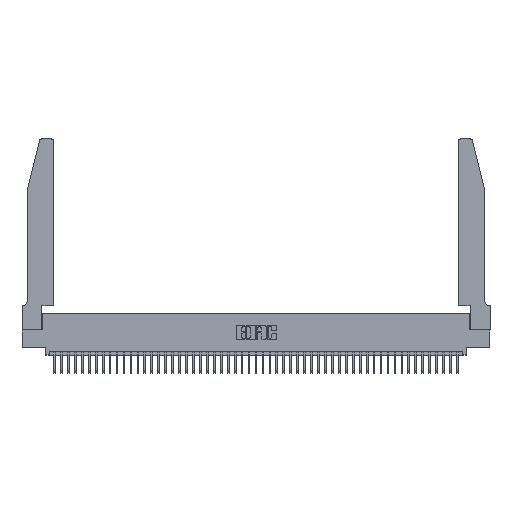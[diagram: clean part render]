
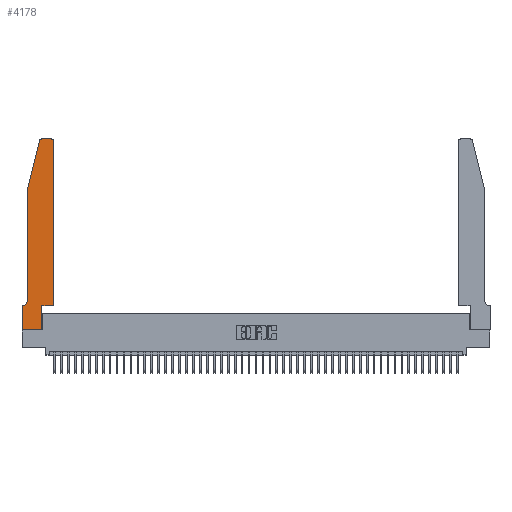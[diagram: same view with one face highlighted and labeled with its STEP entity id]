
A CAD part, top view. The second image highlights one B-rep face of the part: STEP entity #4178.
In plain terms, the highlighted planar face has unit normal (0, 0, 1).
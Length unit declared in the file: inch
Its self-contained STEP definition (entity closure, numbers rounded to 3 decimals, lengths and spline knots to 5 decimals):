
#5 = EDGE_LOOP ( 'NONE', ( #31108, #38971, #48633, #9396, #12701, #38850, #44825, #49659, #22916, #21874, #20541, #32753 ) ) ;
#1253 = VERTEX_POINT ( 'NONE', #48712 ) ;
#2338 = DIRECTION ( 'NONE',  ( 0., 0., -1. ) ) ;
#3318 = CARTESIAN_POINT ( 'NONE',  ( 0.0755, 2., 0.37 ) ) ;
#3496 = AXIS2_PLACEMENT_3D ( 'NONE', #46667, #46176, #20033 ) ;
#4178 = ADVANCED_FACE ( 'NONE', ( #18619 ), #47686, .T. ) ;
#4203 = DIRECTION ( 'NONE',  ( 0., -1., 0. ) ) ;
#4557 = VERTEX_POINT ( 'NONE', #26676 ) ;
#5245 = CARTESIAN_POINT ( 'NONE',  ( 0.25487, 2.72718, 0.37 ) ) ;
#5362 = LINE ( 'NONE', #15091, #50573 ) ;
#5391 = VERTEX_POINT ( 'NONE', #5245 ) ;
#5493 = CARTESIAN_POINT ( 'NONE',  ( 0., 0., 0.37 ) ) ;
#5517 = EDGE_CURVE ( 'NONE', #38527, #18075, #36779, .T. ) ;
#5591 = VECTOR ( 'NONE', #48440, 39.37008 ) ;
#6948 = LINE ( 'NONE', #45353, #34970 ) ;
#7301 = EDGE_CURVE ( 'NONE', #40261, #5391, #34787, .T. ) ;
#8132 = CARTESIAN_POINT ( 'NONE',  ( 0.0755, 2., 0.37 ) ) ;
#8458 = CARTESIAN_POINT ( 'NONE',  ( 0., 0.35, 0.37 ) ) ;
#9337 = VECTOR ( 'NONE', #25352, 39.37008 ) ;
#9396 = ORIENTED_EDGE ( 'NONE', *, *, #14602, .T. ) ;
#9519 = DIRECTION ( 'NONE',  ( -1., 0., 0. ) ) ;
#9538 = VECTOR ( 'NONE', #47108, 39.37008 ) ;
#10536 = DIRECTION ( 'NONE',  ( 1., 0., 0. ) ) ;
#12701 = ORIENTED_EDGE ( 'NONE', *, *, #5517, .T. ) ;
#13118 = LINE ( 'NONE', #46714, #46727 ) ;
#14443 = CARTESIAN_POINT ( 'NONE',  ( 0.284, 2.75, 0.37 ) ) ;
#14602 = EDGE_CURVE ( 'NONE', #28823, #38527, #18881, .T. ) ;
#15091 = CARTESIAN_POINT ( 'NONE',  ( 0.0755, 2., 0.37 ) ) ;
#15298 = LINE ( 'NONE', #22449, #39741 ) ;
#15403 = LINE ( 'NONE', #21926, #9337 ) ;
#15784 = VECTOR ( 'NONE', #4203, 39.37008 ) ;
#17063 = CARTESIAN_POINT ( 'NONE',  ( 0.4505, 2.72, 0.37 ) ) ;
#17135 = EDGE_CURVE ( 'NONE', #18075, #33438, #28187, .T. ) ;
#17838 = DIRECTION ( 'NONE',  ( 1., 0., 0. ) ) ;
#18075 = VERTEX_POINT ( 'NONE', #36444 ) ;
#18619 = FACE_OUTER_BOUND ( 'NONE', #5, .T. ) ;
#18881 = LINE ( 'NONE', #8132, #15784 ) ;
#18951 = CARTESIAN_POINT ( 'NONE',  ( 0.0755, 0.35, 0.37 ) ) ;
#19025 = AXIS2_PLACEMENT_3D ( 'NONE', #8458, #24304, #28271 ) ;
#20033 = DIRECTION ( 'NONE',  ( 1., 0., 0. ) ) ;
#20541 = ORIENTED_EDGE ( 'NONE', *, *, #28687, .T. ) ;
#21041 = VERTEX_POINT ( 'NONE', #5493 ) ;
#21874 = ORIENTED_EDGE ( 'NONE', *, *, #42524, .T. ) ;
#21926 = CARTESIAN_POINT ( 'NONE',  ( 0.4505, 0.35, 0.37 ) ) ;
#21927 = EDGE_CURVE ( 'NONE', #21041, #1253, #6948, .T. ) ;
#22205 = CIRCLE ( 'NONE', #3496, 0.03 ) ;
#22449 = CARTESIAN_POINT ( 'NONE',  ( 0.2605, 2.75, 0.37 ) ) ;
#22916 = ORIENTED_EDGE ( 'NONE', *, *, #46537, .T. ) ;
#23075 = AXIS2_PLACEMENT_3D ( 'NONE', #44815, #44995, #17838 ) ;
#24304 = DIRECTION ( 'NONE',  ( 0., 0., 1. ) ) ;
#24861 = CARTESIAN_POINT ( 'NONE',  ( 0.4505, 0.35, 0.37 ) ) ;
#25035 = CARTESIAN_POINT ( 'NONE',  ( 0.0755, 0.42, 0.37 ) ) ;
#25352 = DIRECTION ( 'NONE',  ( 0., 1., 0. ) ) ;
#25389 = LINE ( 'NONE', #39883, #9538 ) ;
#26562 = DIRECTION ( 'NONE',  ( -0.239, -0.971, 0. ) ) ;
#26676 = CARTESIAN_POINT ( 'NONE',  ( 0.2865, 0.35, 0.37 ) ) ;
#28187 = LINE ( 'NONE', #18951, #45869 ) ;
#28271 = DIRECTION ( 'NONE',  ( 1., 0., 0. ) ) ;
#28687 = EDGE_CURVE ( 'NONE', #42014, #42179, #15403, .T. ) ;
#28823 = VERTEX_POINT ( 'NONE', #3318 ) ;
#29158 = CARTESIAN_POINT ( 'NONE',  ( 0.0055, 0.42, 0.37 ) ) ;
#31108 = ORIENTED_EDGE ( 'NONE', *, *, #42598, .T. ) ;
#32753 = ORIENTED_EDGE ( 'NONE', *, *, #38944, .T. ) ;
#33438 = VERTEX_POINT ( 'NONE', #47121 ) ;
#33977 = EDGE_CURVE ( 'NONE', #33438, #21041, #13118, .T. ) ;
#34699 = VERTEX_POINT ( 'NONE', #46305 ) ;
#34787 = CIRCLE ( 'NONE', #23075, 0.03 ) ;
#34970 = VECTOR ( 'NONE', #10536, 39.37008 ) ;
#35912 = EDGE_CURVE ( 'NONE', #5391, #28823, #5362, .T. ) ;
#36207 = AXIS2_PLACEMENT_3D ( 'NONE', #29158, #2338, #9519 ) ;
#36444 = CARTESIAN_POINT ( 'NONE',  ( 0.0055, 0.35, 0.37 ) ) ;
#36779 = CIRCLE ( 'NONE', #36207, 0.07 ) ;
#38527 = VERTEX_POINT ( 'NONE', #25035 ) ;
#38850 = ORIENTED_EDGE ( 'NONE', *, *, #17135, .T. ) ;
#38944 = EDGE_CURVE ( 'NONE', #42179, #34699, #22205, .T. ) ;
#38971 = ORIENTED_EDGE ( 'NONE', *, *, #7301, .T. ) ;
#39741 = VECTOR ( 'NONE', #45174, 39.37008 ) ;
#39883 = CARTESIAN_POINT ( 'NONE',  ( 0.2865, 0.35, 0.37 ) ) ;
#40261 = VERTEX_POINT ( 'NONE', #14443 ) ;
#41446 = CARTESIAN_POINT ( 'NONE',  ( 0.4505, 0.35, 0.37 ) ) ;
#42014 = VERTEX_POINT ( 'NONE', #41446 ) ;
#42179 = VERTEX_POINT ( 'NONE', #17063 ) ;
#42524 = EDGE_CURVE ( 'NONE', #4557, #42014, #48365, .T. ) ;
#42598 = EDGE_CURVE ( 'NONE', #34699, #40261, #15298, .T. ) ;
#44815 = CARTESIAN_POINT ( 'NONE',  ( 0.284, 2.72, 0.37 ) ) ;
#44825 = ORIENTED_EDGE ( 'NONE', *, *, #33977, .T. ) ;
#44995 = DIRECTION ( 'NONE',  ( 0., 0., 1. ) ) ;
#45174 = DIRECTION ( 'NONE',  ( -1., 0., 0. ) ) ;
#45353 = CARTESIAN_POINT ( 'NONE',  ( 0., 0., 0.37 ) ) ;
#45869 = VECTOR ( 'NONE', #45936, 39.37008 ) ;
#45936 = DIRECTION ( 'NONE',  ( -1., 0., 0. ) ) ;
#46176 = DIRECTION ( 'NONE',  ( 0., 0., 1. ) ) ;
#46305 = CARTESIAN_POINT ( 'NONE',  ( 0.4205, 2.75, 0.37 ) ) ;
#46537 = EDGE_CURVE ( 'NONE', #1253, #4557, #25389, .T. ) ;
#46667 = CARTESIAN_POINT ( 'NONE',  ( 0.4205, 2.72, 0.37 ) ) ;
#46714 = CARTESIAN_POINT ( 'NONE',  ( 0., 0., 0.37 ) ) ;
#46727 = VECTOR ( 'NONE', #46889, 39.37008 ) ;
#46889 = DIRECTION ( 'NONE',  ( 0., -1., 0. ) ) ;
#47108 = DIRECTION ( 'NONE',  ( 0., 1., 0. ) ) ;
#47121 = CARTESIAN_POINT ( 'NONE',  ( 0., 0.35, 0.37 ) ) ;
#47686 = PLANE ( 'NONE',  #19025 ) ;
#48365 = LINE ( 'NONE', #24861, #5591 ) ;
#48440 = DIRECTION ( 'NONE',  ( 1., 0., 0. ) ) ;
#48633 = ORIENTED_EDGE ( 'NONE', *, *, #35912, .T. ) ;
#48712 = CARTESIAN_POINT ( 'NONE',  ( 0.2865, 0., 0.37 ) ) ;
#49659 = ORIENTED_EDGE ( 'NONE', *, *, #21927, .T. ) ;
#50573 = VECTOR ( 'NONE', #26562, 39.37008 ) ;
